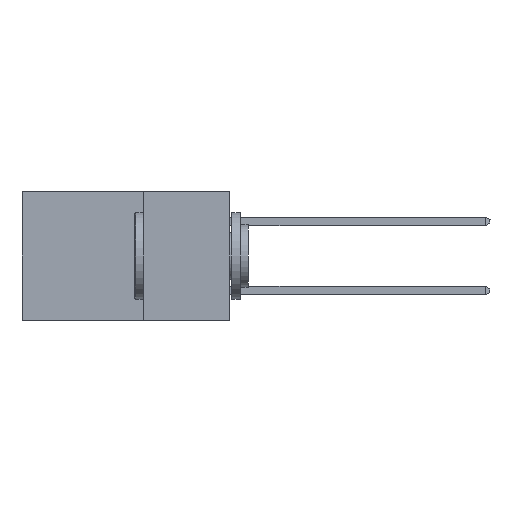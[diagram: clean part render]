
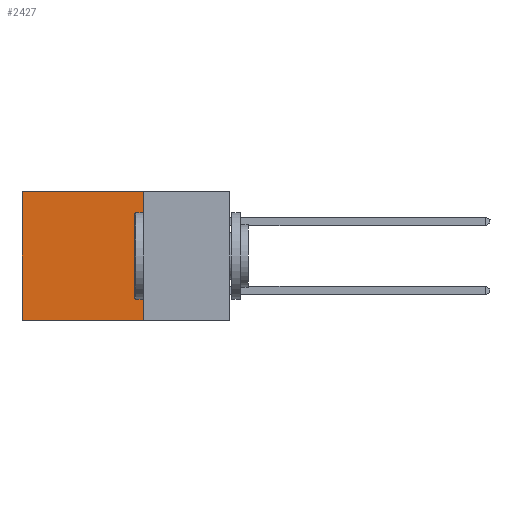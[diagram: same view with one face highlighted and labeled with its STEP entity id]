
A CAD part, left-side view. The second image highlights one B-rep face of the part: STEP entity #2427.
In plain terms, the highlighted planar face has unit normal (-1, 0, 0).
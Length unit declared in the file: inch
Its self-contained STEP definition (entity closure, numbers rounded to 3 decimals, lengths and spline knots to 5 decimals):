
#178 = DIRECTION ( 'NONE',  ( 0., 1., 0. ) ) ;
#433 = DIRECTION ( 'NONE',  ( 1., 0., 0. ) ) ;
#609 = ORIENTED_EDGE ( 'NONE', *, *, #16237, .F. ) ;
#1111 = DIRECTION ( 'NONE',  ( 0., 0., -1. ) ) ;
#2427 = ADVANCED_FACE ( 'NONE', ( #6416 ), #14014, .F. ) ;
#2883 = CARTESIAN_POINT ( 'NONE',  ( 0.298, 0.25, -0.37 ) ) ;
#4773 = LINE ( 'NONE', #2883, #7065 ) ;
#5568 = CARTESIAN_POINT ( 'NONE',  ( 0.298, 0.25, 0. ) ) ;
#5890 = CARTESIAN_POINT ( 'NONE',  ( 0.298, 0.25, -0.37 ) ) ;
#6254 = ORIENTED_EDGE ( 'NONE', *, *, #8482, .T. ) ;
#6416 = FACE_OUTER_BOUND ( 'NONE', #8751, .T. ) ;
#6909 = LINE ( 'NONE', #5568, #7565 ) ;
#7065 = VECTOR ( 'NONE', #8078, 39.37008 ) ;
#7565 = VECTOR ( 'NONE', #178, 39.37008 ) ;
#8065 = LINE ( 'NONE', #14926, #10602 ) ;
#8078 = DIRECTION ( 'NONE',  ( 0., 1., 0. ) ) ;
#8211 = LINE ( 'NONE', #17043, #16755 ) ;
#8482 = EDGE_CURVE ( 'NONE', #15290, #11703, #8065, .T. ) ;
#8751 = EDGE_LOOP ( 'NONE', ( #6254, #609, #9572, #13399 ) ) ;
#9572 = ORIENTED_EDGE ( 'NONE', *, *, #9862, .F. ) ;
#9862 = EDGE_CURVE ( 'NONE', #10728, #10693, #8211, .T. ) ;
#9898 = DIRECTION ( 'NONE',  ( 0., 0., -1. ) ) ;
#10602 = VECTOR ( 'NONE', #13641, 39.37008 ) ;
#10693 = VERTEX_POINT ( 'NONE', #5890 ) ;
#10728 = VERTEX_POINT ( 'NONE', #14090 ) ;
#11703 = VERTEX_POINT ( 'NONE', #11724 ) ;
#11724 = CARTESIAN_POINT ( 'NONE',  ( 0.298, 0.6, -0.37 ) ) ;
#13399 = ORIENTED_EDGE ( 'NONE', *, *, #14929, .T. ) ;
#13641 = DIRECTION ( 'NONE',  ( 0., 0., -1. ) ) ;
#14014 = PLANE ( 'NONE',  #16648 ) ;
#14090 = CARTESIAN_POINT ( 'NONE',  ( 0.298, 0.25, 0. ) ) ;
#14926 = CARTESIAN_POINT ( 'NONE',  ( 0.298, 0.6, 0. ) ) ;
#14929 = EDGE_CURVE ( 'NONE', #10728, #15290, #6909, .T. ) ;
#15290 = VERTEX_POINT ( 'NONE', #16227 ) ;
#16227 = CARTESIAN_POINT ( 'NONE',  ( 0.298, 0.6, 0. ) ) ;
#16237 = EDGE_CURVE ( 'NONE', #10693, #11703, #4773, .T. ) ;
#16648 = AXIS2_PLACEMENT_3D ( 'NONE', #16775, #433, #9898 ) ;
#16755 = VECTOR ( 'NONE', #1111, 39.37008 ) ;
#16775 = CARTESIAN_POINT ( 'NONE',  ( 0.298, 0.25, 0. ) ) ;
#17043 = CARTESIAN_POINT ( 'NONE',  ( 0.298, 0.25, 0. ) ) ;
